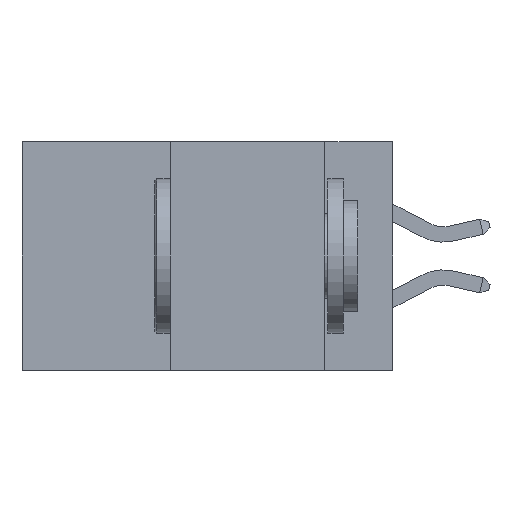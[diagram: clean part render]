
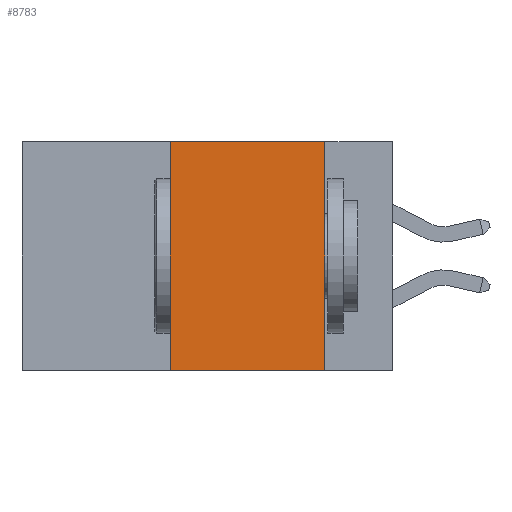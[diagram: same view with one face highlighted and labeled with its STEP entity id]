
A CAD part, left-side view. The second image highlights one B-rep face of the part: STEP entity #8783.
In plain terms, the highlighted planar face has unit normal (-1, 0, 0).
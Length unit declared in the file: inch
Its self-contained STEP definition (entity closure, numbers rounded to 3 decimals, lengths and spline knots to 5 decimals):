
#404 = LINE ( 'NONE', #2699, #13251 ) ;
#450 = AXIS2_PLACEMENT_3D ( 'NONE', #2789, #11713, #4091 ) ;
#1030 = VERTEX_POINT ( 'NONE', #4454 ) ;
#1199 = CARTESIAN_POINT ( 'NONE',  ( 0., 0.11, 0. ) ) ;
#2366 = EDGE_CURVE ( 'NONE', #16003, #1030, #14367, .T. ) ;
#2699 = CARTESIAN_POINT ( 'NONE',  ( 0., 0.36, 0. ) ) ;
#2789 = CARTESIAN_POINT ( 'NONE',  ( 0., 0.6, 0. ) ) ;
#3893 = ORIENTED_EDGE ( 'NONE', *, *, #15434, .F. ) ;
#4033 = PLANE ( 'NONE',  #450 ) ;
#4091 = DIRECTION ( 'NONE',  ( 0., 0., -1. ) ) ;
#4454 = CARTESIAN_POINT ( 'NONE',  ( 0., 0.11, -0.37 ) ) ;
#5256 = EDGE_CURVE ( 'NONE', #15837, #1030, #9971, .T. ) ;
#6026 = EDGE_CURVE ( 'NONE', #8530, #16003, #9823, .T. ) ;
#6133 = FACE_OUTER_BOUND ( 'NONE', #13050, .T. ) ;
#6152 = VECTOR ( 'NONE', #11303, 39.37008 ) ;
#6912 = ORIENTED_EDGE ( 'NONE', *, *, #2366, .F. ) ;
#7707 = CARTESIAN_POINT ( 'NONE',  ( 0., 0.11, 0. ) ) ;
#7860 = DIRECTION ( 'NONE',  ( 0., 0., -1. ) ) ;
#8507 = CARTESIAN_POINT ( 'NONE',  ( 0., 0.36, 0. ) ) ;
#8530 = VERTEX_POINT ( 'NONE', #8507 ) ;
#8783 = ADVANCED_FACE ( 'NONE', ( #6133 ), #4033, .F. ) ;
#9014 = VECTOR ( 'NONE', #11748, 39.37008 ) ;
#9135 = DIRECTION ( 'NONE',  ( 0., 0., 1. ) ) ;
#9823 = LINE ( 'NONE', #10499, #9014 ) ;
#9971 = LINE ( 'NONE', #13877, #6152 ) ;
#10499 = CARTESIAN_POINT ( 'NONE',  ( 0., 0.6, 0. ) ) ;
#11105 = ORIENTED_EDGE ( 'NONE', *, *, #5256, .T. ) ;
#11303 = DIRECTION ( 'NONE',  ( 0., -1., 0. ) ) ;
#11713 = DIRECTION ( 'NONE',  ( 1., 0., 0. ) ) ;
#11748 = DIRECTION ( 'NONE',  ( 0., -1., 0. ) ) ;
#12369 = CARTESIAN_POINT ( 'NONE',  ( 0., 0.36, -0.37 ) ) ;
#13050 = EDGE_LOOP ( 'NONE', ( #6912, #13704, #3893, #11105 ) ) ;
#13215 = VECTOR ( 'NONE', #7860, 39.37008 ) ;
#13251 = VECTOR ( 'NONE', #9135, 39.37008 ) ;
#13704 = ORIENTED_EDGE ( 'NONE', *, *, #6026, .F. ) ;
#13877 = CARTESIAN_POINT ( 'NONE',  ( 0., 0.6, -0.37 ) ) ;
#14367 = LINE ( 'NONE', #7707, #13215 ) ;
#15434 = EDGE_CURVE ( 'NONE', #15837, #8530, #404, .T. ) ;
#15837 = VERTEX_POINT ( 'NONE', #12369 ) ;
#16003 = VERTEX_POINT ( 'NONE', #1199 ) ;
